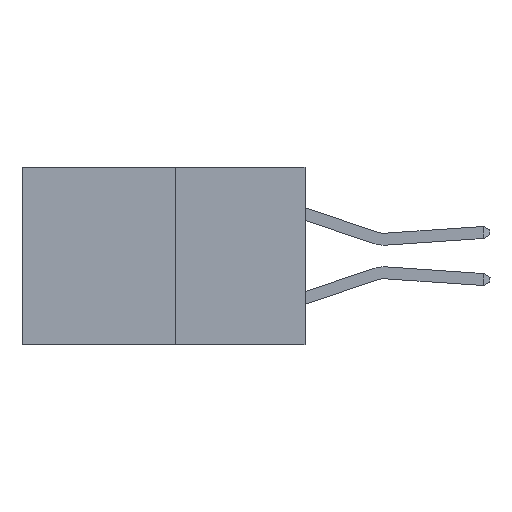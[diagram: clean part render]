
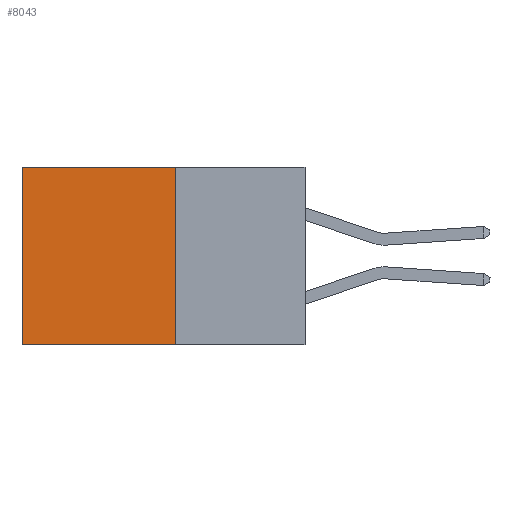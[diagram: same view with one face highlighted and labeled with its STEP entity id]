
A CAD part, left-side view. The second image highlights one B-rep face of the part: STEP entity #8043.
In plain terms, the highlighted planar face has unit normal (-1, 0, 0).
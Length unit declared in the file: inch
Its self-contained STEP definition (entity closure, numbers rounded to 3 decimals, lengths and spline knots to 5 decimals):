
#826 = VERTEX_POINT ( 'NONE', #23451 ) ;
#1738 = PLANE ( 'NONE',  #6236 ) ;
#3095 = VECTOR ( 'NONE', #21861, 39.37008 ) ;
#3775 = FACE_OUTER_BOUND ( 'NONE', #9845, .T. ) ;
#3929 = DIRECTION ( 'NONE',  ( 0., 0., -1. ) ) ;
#6207 = CARTESIAN_POINT ( 'NONE',  ( 0.277, 0.27, -0.37 ) ) ;
#6236 = AXIS2_PLACEMENT_3D ( 'NONE', #6207, #20991, #8382 ) ;
#7630 = EDGE_CURVE ( 'NONE', #19396, #27067, #13920, .T. ) ;
#7742 = DIRECTION ( 'NONE',  ( 0., 1., 0. ) ) ;
#8043 = ADVANCED_FACE ( 'NONE', ( #3775 ), #1738, .F. ) ;
#8244 = ORIENTED_EDGE ( 'NONE', *, *, #12944, .F. ) ;
#8382 = DIRECTION ( 'NONE',  ( 0., 0., -1. ) ) ;
#8740 = EDGE_CURVE ( 'NONE', #826, #8962, #10014, .T. ) ;
#8962 = VERTEX_POINT ( 'NONE', #19450 ) ;
#9251 = CARTESIAN_POINT ( 'NONE',  ( 0.277, 0.59, -0.37 ) ) ;
#9554 = ORIENTED_EDGE ( 'NONE', *, *, #8740, .F. ) ;
#9845 = EDGE_LOOP ( 'NONE', ( #21435, #8244, #9554, #13884 ) ) ;
#10014 = LINE ( 'NONE', #18818, #20518 ) ;
#11171 = LINE ( 'NONE', #26700, #16039 ) ;
#12416 = CARTESIAN_POINT ( 'NONE',  ( 0.277, 0.59, -0.37 ) ) ;
#12944 = EDGE_CURVE ( 'NONE', #8962, #27067, #11171, .T. ) ;
#13019 = EDGE_CURVE ( 'NONE', #826, #19396, #26023, .T. ) ;
#13884 = ORIENTED_EDGE ( 'NONE', *, *, #13019, .T. ) ;
#13920 = LINE ( 'NONE', #9251, #3095 ) ;
#14312 = DIRECTION ( 'NONE',  ( 0., 1., 0. ) ) ;
#16039 = VECTOR ( 'NONE', #7742, 39.37008 ) ;
#18818 = CARTESIAN_POINT ( 'NONE',  ( 0.277, 0.27, -0.37 ) ) ;
#19396 = VERTEX_POINT ( 'NONE', #27447 ) ;
#19450 = CARTESIAN_POINT ( 'NONE',  ( 0.277, 0.27, -0.37 ) ) ;
#20518 = VECTOR ( 'NONE', #3929, 39.37008 ) ;
#20991 = DIRECTION ( 'NONE',  ( 1., 0., 0. ) ) ;
#21435 = ORIENTED_EDGE ( 'NONE', *, *, #7630, .T. ) ;
#21674 = VECTOR ( 'NONE', #14312, 39.37008 ) ;
#21861 = DIRECTION ( 'NONE',  ( 0., 0., -1. ) ) ;
#23451 = CARTESIAN_POINT ( 'NONE',  ( 0.277, 0.27, 0. ) ) ;
#26023 = LINE ( 'NONE', #26976, #21674 ) ;
#26700 = CARTESIAN_POINT ( 'NONE',  ( 0.277, 0.27, -0.37 ) ) ;
#26976 = CARTESIAN_POINT ( 'NONE',  ( 0.277, 0.27, 0. ) ) ;
#27067 = VERTEX_POINT ( 'NONE', #12416 ) ;
#27447 = CARTESIAN_POINT ( 'NONE',  ( 0.277, 0.59, 0. ) ) ;
